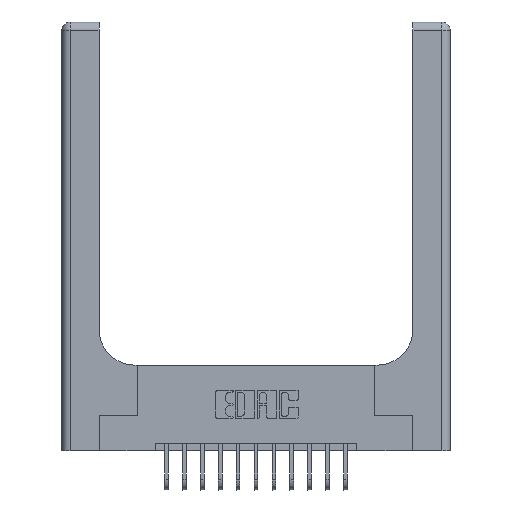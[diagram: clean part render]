
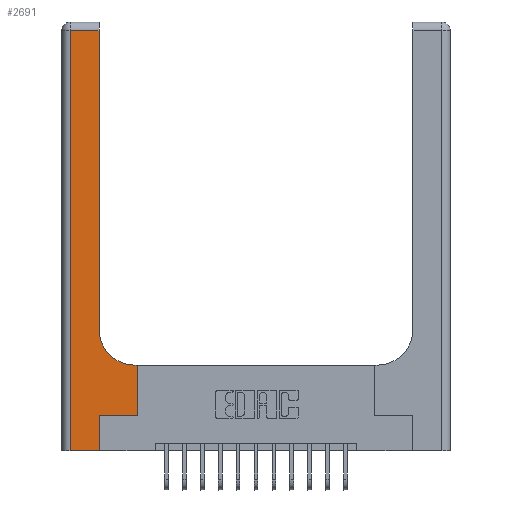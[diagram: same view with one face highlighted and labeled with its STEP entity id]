
A CAD part, top view. The second image highlights one B-rep face of the part: STEP entity #2691.
In plain terms, the highlighted planar face has unit normal (0, 0, 1).
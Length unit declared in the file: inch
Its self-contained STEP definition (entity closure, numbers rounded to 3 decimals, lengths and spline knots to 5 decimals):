
#43 = VECTOR ( 'NONE', #9419, 39.37008 ) ;
#249 = VERTEX_POINT ( 'NONE', #5635 ) ;
#779 = CARTESIAN_POINT ( 'NONE',  ( 0.528, 0.25, 0.37 ) ) ;
#1035 = EDGE_CURVE ( 'NONE', #249, #5998, #13428, .T. ) ;
#1038 = ORIENTED_EDGE ( 'NONE', *, *, #3035, .T. ) ;
#1348 = CARTESIAN_POINT ( 'NONE',  ( 0.26, 0.85, 0.37 ) ) ;
#1370 = VERTEX_POINT ( 'NONE', #8681 ) ;
#1605 = ORIENTED_EDGE ( 'NONE', *, *, #16038, .T. ) ;
#2028 = VERTEX_POINT ( 'NONE', #1348 ) ;
#2217 = VERTEX_POINT ( 'NONE', #13013 ) ;
#2381 = ORIENTED_EDGE ( 'NONE', *, *, #14787, .T. ) ;
#2488 = DIRECTION ( 'NONE',  ( -1., 0., 0. ) ) ;
#2500 = DIRECTION ( 'NONE',  ( 0., 0., -1. ) ) ;
#2542 = VECTOR ( 'NONE', #12015, 39.37008 ) ;
#2691 = ADVANCED_FACE ( 'NONE', ( #15514 ), #2894, .F. ) ;
#2894 = PLANE ( 'NONE',  #5488 ) ;
#2979 = ORIENTED_EDGE ( 'NONE', *, *, #1035, .T. ) ;
#3034 = LINE ( 'NONE', #6234, #15562 ) ;
#3035 = EDGE_CURVE ( 'NONE', #8926, #2028, #7925, .T. ) ;
#4156 = VECTOR ( 'NONE', #4350, 39.37008 ) ;
#4181 = DIRECTION ( 'NONE',  ( 0., 0., -1. ) ) ;
#4312 = ORIENTED_EDGE ( 'NONE', *, *, #13312, .T. ) ;
#4350 = DIRECTION ( 'NONE',  ( 0., 1., 0. ) ) ;
#5488 = AXIS2_PLACEMENT_3D ( 'NONE', #10444, #4181, #12936 ) ;
#5635 = CARTESIAN_POINT ( 'NONE',  ( 0.06, 0., 0.37 ) ) ;
#5643 = VECTOR ( 'NONE', #15377, 39.37008 ) ;
#5998 = VERTEX_POINT ( 'NONE', #10355 ) ;
#6234 = CARTESIAN_POINT ( 'NONE',  ( 0.265, 0.25, 0.37 ) ) ;
#6284 = CARTESIAN_POINT ( 'NONE',  ( 0.26, 0.6, 0.37 ) ) ;
#6446 = VERTEX_POINT ( 'NONE', #779 ) ;
#6878 = AXIS2_PLACEMENT_3D ( 'NONE', #10055, #2500, #11317 ) ;
#6905 = CARTESIAN_POINT ( 'NONE',  ( 0., 0., 0.37 ) ) ;
#7544 = VECTOR ( 'NONE', #8582, 39.37008 ) ;
#7925 = CIRCLE ( 'NONE', #6878, 0.25 ) ;
#8582 = DIRECTION ( 'NONE',  ( 0., 1., 0. ) ) ;
#8610 = EDGE_CURVE ( 'NONE', #16146, #15068, #14821, .T. ) ;
#8681 = CARTESIAN_POINT ( 'NONE',  ( 0.528, 0.6, 0.37 ) ) ;
#8926 = VERTEX_POINT ( 'NONE', #11323 ) ;
#9316 = CARTESIAN_POINT ( 'NONE',  ( 0., 2.94, 0.37 ) ) ;
#9419 = DIRECTION ( 'NONE',  ( 1., 0., 0. ) ) ;
#10055 = CARTESIAN_POINT ( 'NONE',  ( 0.51, 0.85, 0.37 ) ) ;
#10355 = CARTESIAN_POINT ( 'NONE',  ( 0.265, 0., 0.37 ) ) ;
#10444 = CARTESIAN_POINT ( 'NONE',  ( 0., 3., 0.37 ) ) ;
#10449 = CARTESIAN_POINT ( 'NONE',  ( 0.06, 3., 0.37 ) ) ;
#10772 = CARTESIAN_POINT ( 'NONE',  ( 0.26, 3., 0.37 ) ) ;
#10833 = LINE ( 'NONE', #11858, #4156 ) ;
#10864 = LINE ( 'NONE', #13534, #7544 ) ;
#11125 = ORIENTED_EDGE ( 'NONE', *, *, #14364, .T. ) ;
#11317 = DIRECTION ( 'NONE',  ( 1., 0., 0. ) ) ;
#11323 = CARTESIAN_POINT ( 'NONE',  ( 0.51, 0.6, 0.37 ) ) ;
#11694 = EDGE_LOOP ( 'NONE', ( #12942, #12499, #11125, #2979, #1605, #2381, #4312, #12852, #1038 ) ) ;
#11858 = CARTESIAN_POINT ( 'NONE',  ( 0.528, 0.25, 0.37 ) ) ;
#11952 = EDGE_CURVE ( 'NONE', #1370, #8926, #12790, .T. ) ;
#12015 = DIRECTION ( 'NONE',  ( 0., 1., 0. ) ) ;
#12272 = LINE ( 'NONE', #10449, #5643 ) ;
#12499 = ORIENTED_EDGE ( 'NONE', *, *, #8610, .T. ) ;
#12571 = LINE ( 'NONE', #10772, #2542 ) ;
#12790 = LINE ( 'NONE', #6284, #13185 ) ;
#12852 = ORIENTED_EDGE ( 'NONE', *, *, #11952, .T. ) ;
#12876 = CARTESIAN_POINT ( 'NONE',  ( 0.06, 2.94, 0.37 ) ) ;
#12936 = DIRECTION ( 'NONE',  ( -1., 0., 0. ) ) ;
#12942 = ORIENTED_EDGE ( 'NONE', *, *, #13383, .T. ) ;
#13013 = CARTESIAN_POINT ( 'NONE',  ( 0.265, 0.25, 0.37 ) ) ;
#13185 = VECTOR ( 'NONE', #2488, 39.37008 ) ;
#13312 = EDGE_CURVE ( 'NONE', #6446, #1370, #10833, .T. ) ;
#13383 = EDGE_CURVE ( 'NONE', #2028, #16146, #12571, .T. ) ;
#13428 = LINE ( 'NONE', #6905, #43 ) ;
#13534 = CARTESIAN_POINT ( 'NONE',  ( 0.265, 0., 0.37 ) ) ;
#14056 = VECTOR ( 'NONE', #14520, 39.37008 ) ;
#14364 = EDGE_CURVE ( 'NONE', #15068, #249, #12272, .T. ) ;
#14520 = DIRECTION ( 'NONE',  ( -1., 0., 0. ) ) ;
#14787 = EDGE_CURVE ( 'NONE', #2217, #6446, #3034, .T. ) ;
#14821 = LINE ( 'NONE', #9316, #14056 ) ;
#14948 = CARTESIAN_POINT ( 'NONE',  ( 0.26, 2.94, 0.37 ) ) ;
#15068 = VERTEX_POINT ( 'NONE', #12876 ) ;
#15377 = DIRECTION ( 'NONE',  ( 0., -1., 0. ) ) ;
#15514 = FACE_OUTER_BOUND ( 'NONE', #11694, .T. ) ;
#15562 = VECTOR ( 'NONE', #16181, 39.37008 ) ;
#16038 = EDGE_CURVE ( 'NONE', #5998, #2217, #10864, .T. ) ;
#16146 = VERTEX_POINT ( 'NONE', #14948 ) ;
#16181 = DIRECTION ( 'NONE',  ( 1., 0., 0. ) ) ;
